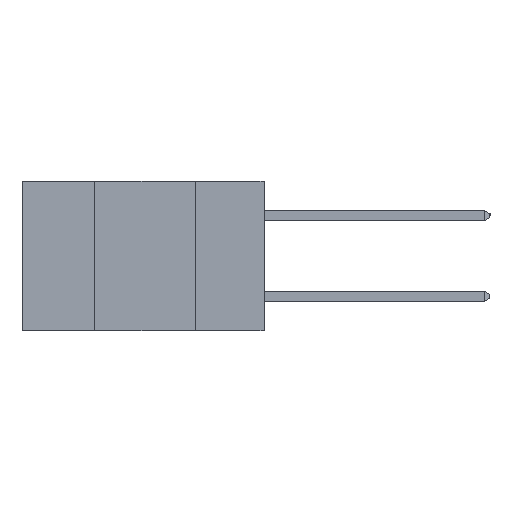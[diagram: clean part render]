
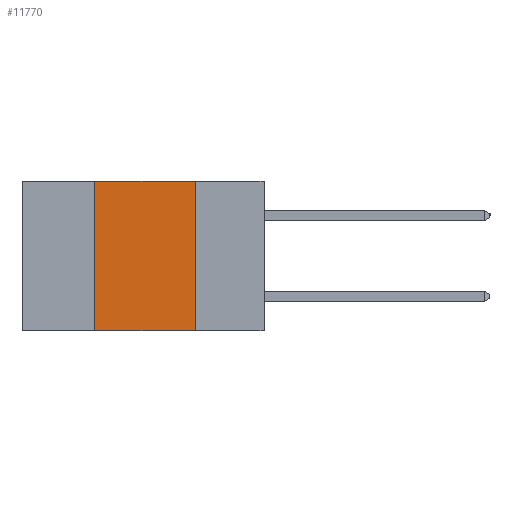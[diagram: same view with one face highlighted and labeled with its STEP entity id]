
A CAD part, left-side view. The second image highlights one B-rep face of the part: STEP entity #11770.
In plain terms, the highlighted planar face has unit normal (-1, 0, 0).
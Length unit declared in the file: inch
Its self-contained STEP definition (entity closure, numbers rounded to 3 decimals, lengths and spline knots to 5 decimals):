
#364 = VECTOR ( 'NONE', #21850, 39.37008 ) ;
#413 = VECTOR ( 'NONE', #13473, 39.37008 ) ;
#1141 = DIRECTION ( 'NONE',  ( 0., 0., -1. ) ) ;
#1438 = CARTESIAN_POINT ( 'NONE',  ( 0., 0.17, -0.37 ) ) ;
#1462 = DIRECTION ( 'NONE',  ( 0., 0., -1. ) ) ;
#1523 = PLANE ( 'NONE',  #2880 ) ;
#2880 = AXIS2_PLACEMENT_3D ( 'NONE', #10911, #16810, #1141 ) ;
#3839 = LINE ( 'NONE', #9109, #413 ) ;
#4659 = VERTEX_POINT ( 'NONE', #7738 ) ;
#5339 = CARTESIAN_POINT ( 'NONE',  ( 0., 0.17, -0.37 ) ) ;
#5457 = ORIENTED_EDGE ( 'NONE', *, *, #5940, .T. ) ;
#5940 = EDGE_CURVE ( 'NONE', #22163, #23566, #12062, .T. ) ;
#6599 = CARTESIAN_POINT ( 'NONE',  ( 0., 0.17, 0. ) ) ;
#6755 = FACE_OUTER_BOUND ( 'NONE', #17886, .T. ) ;
#7738 = CARTESIAN_POINT ( 'NONE',  ( 0., 0.42, 0. ) ) ;
#7873 = VECTOR ( 'NONE', #1462, 39.37008 ) ;
#9109 = CARTESIAN_POINT ( 'NONE',  ( 0., 0.6, 0. ) ) ;
#9351 = EDGE_CURVE ( 'NONE', #22163, #4659, #12143, .T. ) ;
#10911 = CARTESIAN_POINT ( 'NONE',  ( 0., 0.6, 0. ) ) ;
#11105 = ORIENTED_EDGE ( 'NONE', *, *, #19443, .F. ) ;
#11770 = ADVANCED_FACE ( 'NONE', ( #6755 ), #1523, .F. ) ;
#12062 = LINE ( 'NONE', #16102, #14263 ) ;
#12143 = LINE ( 'NONE', #14160, #364 ) ;
#12350 = EDGE_CURVE ( 'NONE', #4659, #18997, #3839, .T. ) ;
#13473 = DIRECTION ( 'NONE',  ( 0., -1., 0. ) ) ;
#14160 = CARTESIAN_POINT ( 'NONE',  ( 0., 0.42, -0.37 ) ) ;
#14263 = VECTOR ( 'NONE', #20115, 39.37008 ) ;
#15879 = ORIENTED_EDGE ( 'NONE', *, *, #9351, .F. ) ;
#16102 = CARTESIAN_POINT ( 'NONE',  ( 0., 0.6, -0.37 ) ) ;
#16400 = ORIENTED_EDGE ( 'NONE', *, *, #12350, .F. ) ;
#16810 = DIRECTION ( 'NONE',  ( 1., 0., 0. ) ) ;
#17886 = EDGE_LOOP ( 'NONE', ( #11105, #16400, #15879, #5457 ) ) ;
#18997 = VERTEX_POINT ( 'NONE', #6599 ) ;
#19443 = EDGE_CURVE ( 'NONE', #18997, #23566, #21013, .T. ) ;
#20115 = DIRECTION ( 'NONE',  ( 0., -1., 0. ) ) ;
#21013 = LINE ( 'NONE', #5339, #7873 ) ;
#21850 = DIRECTION ( 'NONE',  ( 0., 0., 1. ) ) ;
#22163 = VERTEX_POINT ( 'NONE', #24514 ) ;
#23566 = VERTEX_POINT ( 'NONE', #1438 ) ;
#24514 = CARTESIAN_POINT ( 'NONE',  ( 0., 0.42, -0.37 ) ) ;
